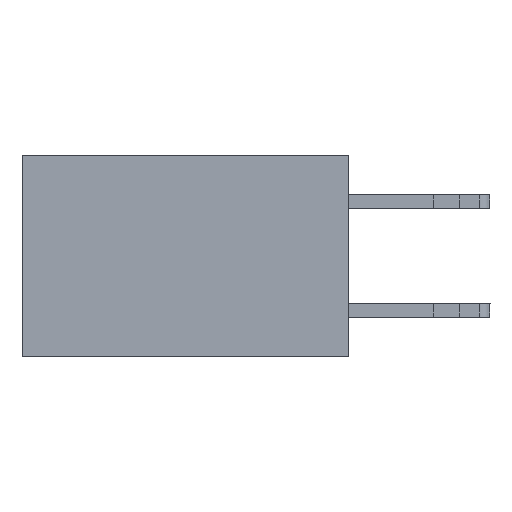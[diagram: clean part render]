
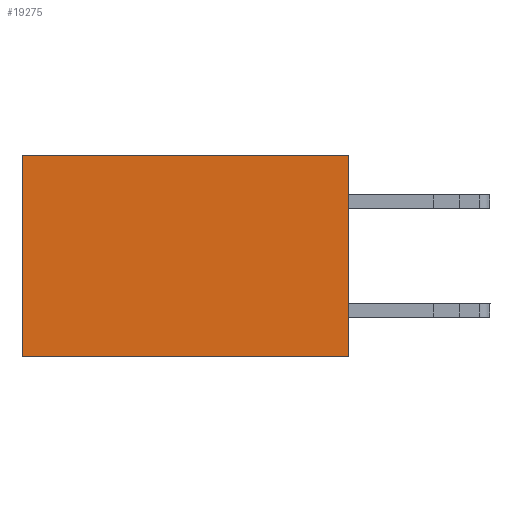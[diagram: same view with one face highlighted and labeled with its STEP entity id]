
A CAD part, left-side view. The second image highlights one B-rep face of the part: STEP entity #19275.
In plain terms, the highlighted planar face has unit normal (-1, 0, 0).
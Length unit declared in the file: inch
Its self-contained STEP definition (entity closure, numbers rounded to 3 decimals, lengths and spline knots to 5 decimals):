
#19 = CARTESIAN_POINT ( 'NONE',  ( 0.298, 0., -0.37 ) ) ;
#207 = VERTEX_POINT ( 'NONE', #11906 ) ;
#463 = DIRECTION ( 'NONE',  ( 1., 0., 0. ) ) ;
#613 = LINE ( 'NONE', #17105, #19036 ) ;
#632 = LINE ( 'NONE', #2514, #19962 ) ;
#2514 = CARTESIAN_POINT ( 'NONE',  ( 0.298, 0., 0. ) ) ;
#2522 = VERTEX_POINT ( 'NONE', #6652 ) ;
#4093 = LINE ( 'NONE', #19742, #9570 ) ;
#4263 = DIRECTION ( 'NONE',  ( 0., 0., -1. ) ) ;
#6066 = VERTEX_POINT ( 'NONE', #23824 ) ;
#6652 = CARTESIAN_POINT ( 'NONE',  ( 0.298, 0.6, 0. ) ) ;
#7426 = ORIENTED_EDGE ( 'NONE', *, *, #19876, .F. ) ;
#7831 = VERTEX_POINT ( 'NONE', #19 ) ;
#8204 = CARTESIAN_POINT ( 'NONE',  ( 0.298, 0., 0. ) ) ;
#8681 = EDGE_CURVE ( 'NONE', #207, #2522, #632, .T. ) ;
#9025 = EDGE_CURVE ( 'NONE', #2522, #6066, #4093, .T. ) ;
#9570 = VECTOR ( 'NONE', #10600, 39.37008 ) ;
#9857 = ORIENTED_EDGE ( 'NONE', *, *, #15006, .F. ) ;
#10600 = DIRECTION ( 'NONE',  ( 0., 0., -1. ) ) ;
#10635 = LINE ( 'NONE', #8204, #16353 ) ;
#11652 = DIRECTION ( 'NONE',  ( 0., 1., 0. ) ) ;
#11906 = CARTESIAN_POINT ( 'NONE',  ( 0.298, 0., 0. ) ) ;
#12179 = FACE_OUTER_BOUND ( 'NONE', #17776, .T. ) ;
#13212 = CARTESIAN_POINT ( 'NONE',  ( 0.298, 0., 0. ) ) ;
#15006 = EDGE_CURVE ( 'NONE', #207, #7831, #10635, .T. ) ;
#16353 = VECTOR ( 'NONE', #21048, 39.37008 ) ;
#16691 = AXIS2_PLACEMENT_3D ( 'NONE', #13212, #463, #4263 ) ;
#16753 = ORIENTED_EDGE ( 'NONE', *, *, #9025, .T. ) ;
#17105 = CARTESIAN_POINT ( 'NONE',  ( 0.298, 0., -0.37 ) ) ;
#17776 = EDGE_LOOP ( 'NONE', ( #16753, #7426, #9857, #23805 ) ) ;
#19036 = VECTOR ( 'NONE', #11652, 39.37008 ) ;
#19275 = ADVANCED_FACE ( 'NONE', ( #12179 ), #22452, .F. ) ;
#19742 = CARTESIAN_POINT ( 'NONE',  ( 0.298, 0.6, 0. ) ) ;
#19876 = EDGE_CURVE ( 'NONE', #7831, #6066, #613, .T. ) ;
#19962 = VECTOR ( 'NONE', #22561, 39.37008 ) ;
#21048 = DIRECTION ( 'NONE',  ( 0., 0., -1. ) ) ;
#22452 = PLANE ( 'NONE',  #16691 ) ;
#22561 = DIRECTION ( 'NONE',  ( 0., 1., 0. ) ) ;
#23805 = ORIENTED_EDGE ( 'NONE', *, *, #8681, .T. ) ;
#23824 = CARTESIAN_POINT ( 'NONE',  ( 0.298, 0.6, -0.37 ) ) ;
